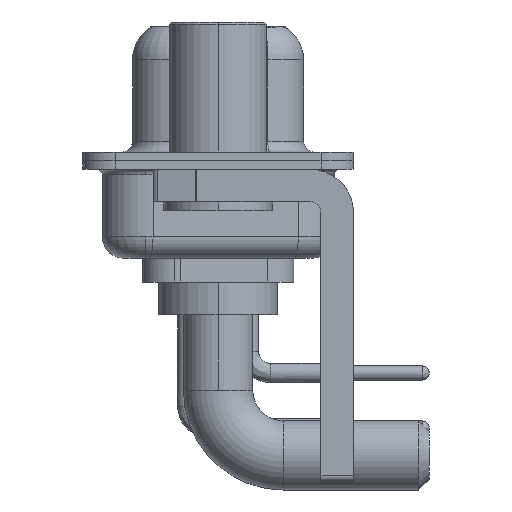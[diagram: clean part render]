
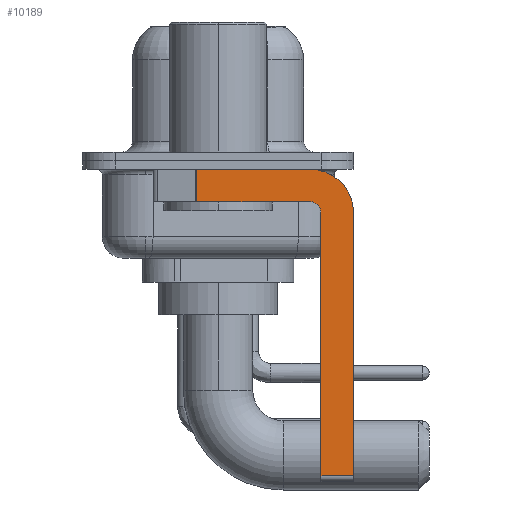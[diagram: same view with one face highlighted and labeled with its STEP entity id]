
A CAD part, left-side view. The second image highlights one B-rep face of the part: STEP entity #10189.
In plain terms, the highlighted planar face has unit normal (-1, 0, 0).
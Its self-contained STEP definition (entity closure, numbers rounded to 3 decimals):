
#90 = DIRECTION ( 'NONE',  ( -1., 0., 0. ) ) ;
#185 = DIRECTION ( 'NONE',  ( 0., -1., 0. ) ) ;
#240 = VERTEX_POINT ( 'NONE', #1096 ) ;
#300 = DIRECTION ( 'NONE',  ( 1., 0., 0. ) ) ;
#402 = CARTESIAN_POINT ( 'NONE',  ( -2.9, -4.25, -2.4 ) ) ;
#1096 = CARTESIAN_POINT ( 'NONE',  ( -2.9, -4.75, -14.55 ) ) ;
#1719 = CARTESIAN_POINT ( 'NONE',  ( -2.9, -6.25, -2.4 ) ) ;
#1887 = LINE ( 'NONE', #6691, #15614 ) ;
#2107 = VECTOR ( 'NONE', #14360, 1000. ) ;
#2532 = CARTESIAN_POINT ( 'NONE',  ( -2.9, 0.978, -1.9 ) ) ;
#2606 = LINE ( 'NONE', #11333, #2107 ) ;
#5100 = FACE_OUTER_BOUND ( 'NONE', #8179, .T. ) ;
#5169 = AXIS2_PLACEMENT_3D ( 'NONE', #402, #300, #20162 ) ;
#5391 = CARTESIAN_POINT ( 'NONE',  ( -2.9, 0.978, -0.4 ) ) ;
#5850 = CARTESIAN_POINT ( 'NONE',  ( -2.9, -4.25, -1.9 ) ) ;
#6211 = EDGE_CURVE ( 'NONE', #20265, #8022, #17178, .T. ) ;
#6547 = VECTOR ( 'NONE', #14156, 1000. ) ;
#6597 = ORIENTED_EDGE ( 'NONE', *, *, #6211, .F. ) ;
#6691 = CARTESIAN_POINT ( 'NONE',  ( -2.9, -4.75, -14.8 ) ) ;
#6897 = VECTOR ( 'NONE', #11575, 1000. ) ;
#7583 = ORIENTED_EDGE ( 'NONE', *, *, #18545, .F. ) ;
#7943 = EDGE_CURVE ( 'NONE', #17546, #10892, #10835, .T. ) ;
#8022 = VERTEX_POINT ( 'NONE', #12567 ) ;
#8179 = EDGE_LOOP ( 'NONE', ( #6597, #19361, #18142, #7583, #17421, #14849, #10760, #14717 ) ) ;
#8540 = DIRECTION ( 'NONE',  ( 0., 0., 1. ) ) ;
#9042 = LINE ( 'NONE', #21056, #6547 ) ;
#10011 = CARTESIAN_POINT ( 'NONE',  ( -2.9, -4.25, -2.4 ) ) ;
#10189 = ADVANCED_FACE ( 'NONE', ( #5100 ), #11958, .F. ) ;
#10253 = VERTEX_POINT ( 'NONE', #1719 ) ;
#10760 = ORIENTED_EDGE ( 'NONE', *, *, #17100, .F. ) ;
#10835 = LINE ( 'NONE', #10956, #11710 ) ;
#10892 = VERTEX_POINT ( 'NONE', #2532 ) ;
#10956 = CARTESIAN_POINT ( 'NONE',  ( -2.9, -4.25, -1.9 ) ) ;
#11333 = CARTESIAN_POINT ( 'NONE',  ( -2.9, -6.25, -2.4 ) ) ;
#11571 = AXIS2_PLACEMENT_3D ( 'NONE', #10011, #90, #16550 ) ;
#11575 = DIRECTION ( 'NONE',  ( 0., -1., 0. ) ) ;
#11710 = VECTOR ( 'NONE', #18019, 1000. ) ;
#11908 = CARTESIAN_POINT ( 'NONE',  ( -2.9, -4.75, -2.4 ) ) ;
#11922 = AXIS2_PLACEMENT_3D ( 'NONE', #13659, #17164, #13764 ) ;
#11958 = PLANE ( 'NONE',  #5169 ) ;
#12076 = EDGE_CURVE ( 'NONE', #240, #13879, #1887, .T. ) ;
#12321 = VECTOR ( 'NONE', #185, 1000. ) ;
#12567 = CARTESIAN_POINT ( 'NONE',  ( -2.9, -4.25, -0.4 ) ) ;
#12708 = VERTEX_POINT ( 'NONE', #13682 ) ;
#13659 = CARTESIAN_POINT ( 'NONE',  ( -2.9, -4.25, -2.4 ) ) ;
#13682 = CARTESIAN_POINT ( 'NONE',  ( -2.9, -6.25, -14.55 ) ) ;
#13764 = DIRECTION ( 'NONE',  ( 0., 0., -1. ) ) ;
#13879 = VERTEX_POINT ( 'NONE', #11908 ) ;
#14156 = DIRECTION ( 'NONE',  ( 0., 0., -1. ) ) ;
#14243 = EDGE_CURVE ( 'NONE', #240, #12708, #14505, .T. ) ;
#14360 = DIRECTION ( 'NONE',  ( 0., 0., -1. ) ) ;
#14505 = LINE ( 'NONE', #21200, #6897 ) ;
#14677 = EDGE_CURVE ( 'NONE', #20265, #10892, #9042, .T. ) ;
#14717 = ORIENTED_EDGE ( 'NONE', *, *, #19109, .F. ) ;
#14849 = ORIENTED_EDGE ( 'NONE', *, *, #14243, .T. ) ;
#15530 = CARTESIAN_POINT ( 'NONE',  ( -2.9, 3., -0.4 ) ) ;
#15614 = VECTOR ( 'NONE', #8540, 1000. ) ;
#16550 = DIRECTION ( 'NONE',  ( 0., 0., 1. ) ) ;
#17100 = EDGE_CURVE ( 'NONE', #10253, #12708, #2606, .T. ) ;
#17164 = DIRECTION ( 'NONE',  ( 1., 0., 0. ) ) ;
#17178 = LINE ( 'NONE', #15530, #12321 ) ;
#17421 = ORIENTED_EDGE ( 'NONE', *, *, #12076, .F. ) ;
#17546 = VERTEX_POINT ( 'NONE', #5850 ) ;
#18019 = DIRECTION ( 'NONE',  ( 0., 1., 0. ) ) ;
#18142 = ORIENTED_EDGE ( 'NONE', *, *, #7943, .F. ) ;
#18545 = EDGE_CURVE ( 'NONE', #13879, #17546, #19246, .T. ) ;
#19109 = EDGE_CURVE ( 'NONE', #8022, #10253, #19259, .T. ) ;
#19246 = CIRCLE ( 'NONE', #11571, 0.5 ) ;
#19259 = CIRCLE ( 'NONE', #11922, 2. ) ;
#19361 = ORIENTED_EDGE ( 'NONE', *, *, #14677, .T. ) ;
#20162 = DIRECTION ( 'NONE',  ( 0., 0., -1. ) ) ;
#20265 = VERTEX_POINT ( 'NONE', #5391 ) ;
#21056 = CARTESIAN_POINT ( 'NONE',  ( -2.9, 0.978, -1.9 ) ) ;
#21200 = CARTESIAN_POINT ( 'NONE',  ( -2.9, -4.25, -14.55 ) ) ;
